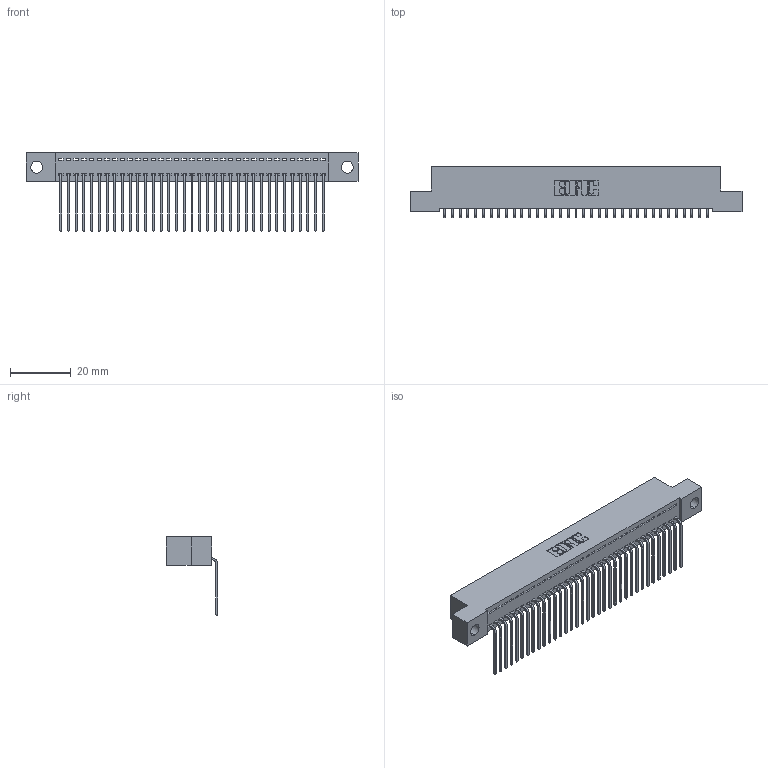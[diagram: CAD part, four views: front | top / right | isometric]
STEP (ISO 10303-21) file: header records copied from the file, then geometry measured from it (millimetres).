
FILE_DESCRIPTION (( 'STEP AP203' ), '1' );
FILE_NAME ('392-035-559-104.STEP', '2019-10-07T16:48:41', ( '' ), ( '' ), 'SwSTEP 2.0', 'SolidWorks 2016', '' );
FILE_SCHEMA (( 'CONFIG_CONTROL_DESIGN' ));
Length unit declared in the file: inch
Products named in the file (3): 345-292-001_558 559 Tail - 1; 392-035-559-104; 342 Part_.156 TH
Assembly tree (36 placements, depth 2):
  392-035-559-104
    342 Part_.156 TH
    345-292-001_558 559 Tail - 1  x35
Bounding box: 109.22 x 16.83 x 25.78 mm (x, y, z)
Volume: 9580.2 mm3; surface area: 14418.5 mm2
Topology: 36 solids, 36 shells, 2210 faces, 6669 edges, 4398 vertices
Faces by surface type: plane 1606, cylinder 604
Entity records: 22257 total; most frequent: CARTESIAN_POINT 3847, ORIENTED_EDGE 3818, DIRECTION 3259, EDGE_CURVE 1909, LINE 1781, VECTOR 1781, VERTEX_POINT 1270, AXIS2_PLACEMENT_3D 739
